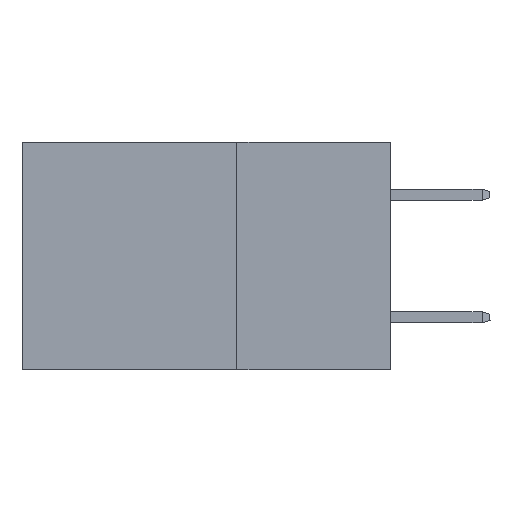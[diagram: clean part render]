
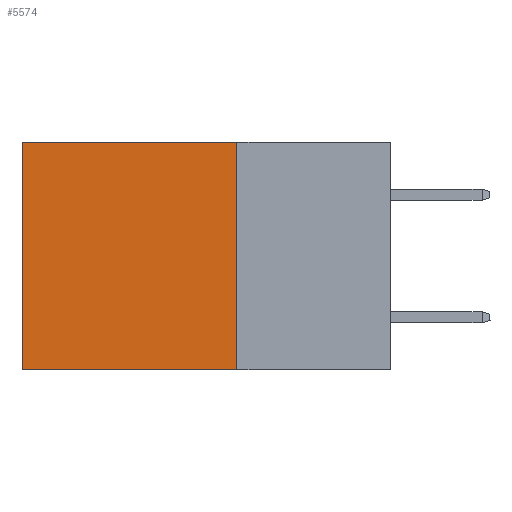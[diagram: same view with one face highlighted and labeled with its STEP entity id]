
A CAD part, left-side view. The second image highlights one B-rep face of the part: STEP entity #5574.
In plain terms, the highlighted planar face has unit normal (-1, 0, 0).
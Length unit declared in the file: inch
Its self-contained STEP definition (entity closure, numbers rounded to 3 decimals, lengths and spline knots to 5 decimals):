
#108 = LINE ( 'NONE', #9904, #724 ) ;
#724 = VECTOR ( 'NONE', #21830, 39.37008 ) ;
#992 = DIRECTION ( 'NONE',  ( 0., 1., 0. ) ) ;
#1916 = EDGE_CURVE ( 'NONE', #11666, #8930, #108, .T. ) ;
#2878 = EDGE_CURVE ( 'NONE', #23693, #8930, #4395, .T. ) ;
#3027 = ORIENTED_EDGE ( 'NONE', *, *, #3966, .F. ) ;
#3966 = EDGE_CURVE ( 'NONE', #14966, #23693, #5213, .T. ) ;
#4370 = EDGE_CURVE ( 'NONE', #14966, #11666, #19266, .T. ) ;
#4395 = LINE ( 'NONE', #18837, #23237 ) ;
#4481 = DIRECTION ( 'NONE',  ( 0., 0., -1. ) ) ;
#4634 = VECTOR ( 'NONE', #19960, 39.37008 ) ;
#5190 = VECTOR ( 'NONE', #992, 39.37008 ) ;
#5213 = LINE ( 'NONE', #11026, #4634 ) ;
#5574 = ADVANCED_FACE ( 'NONE', ( #22275 ), #8252, .F. ) ;
#6654 = CARTESIAN_POINT ( 'NONE',  ( 0.2875, 0.25, 0. ) ) ;
#8252 = PLANE ( 'NONE',  #16529 ) ;
#8254 = CARTESIAN_POINT ( 'NONE',  ( 0.2875, 0.6, -0.37 ) ) ;
#8930 = VERTEX_POINT ( 'NONE', #8254 ) ;
#9017 = CARTESIAN_POINT ( 'NONE',  ( 0.2875, 0.25, -0.37 ) ) ;
#9060 = ORIENTED_EDGE ( 'NONE', *, *, #1916, .T. ) ;
#9904 = CARTESIAN_POINT ( 'NONE',  ( 0.2875, 0.6, 0. ) ) ;
#10482 = EDGE_LOOP ( 'NONE', ( #9060, #11539, #3027, #12369 ) ) ;
#11026 = CARTESIAN_POINT ( 'NONE',  ( 0.2875, 0.25, 0. ) ) ;
#11539 = ORIENTED_EDGE ( 'NONE', *, *, #2878, .F. ) ;
#11666 = VERTEX_POINT ( 'NONE', #19236 ) ;
#12369 = ORIENTED_EDGE ( 'NONE', *, *, #4370, .T. ) ;
#13835 = CARTESIAN_POINT ( 'NONE',  ( 0.2875, 0.25, 0. ) ) ;
#14966 = VERTEX_POINT ( 'NONE', #19986 ) ;
#15626 = DIRECTION ( 'NONE',  ( 1., 0., 0. ) ) ;
#16529 = AXIS2_PLACEMENT_3D ( 'NONE', #13835, #15626, #4481 ) ;
#18837 = CARTESIAN_POINT ( 'NONE',  ( 0.2875, 0.25, -0.37 ) ) ;
#19236 = CARTESIAN_POINT ( 'NONE',  ( 0.2875, 0.6, 0. ) ) ;
#19266 = LINE ( 'NONE', #6654, #5190 ) ;
#19960 = DIRECTION ( 'NONE',  ( 0., 0., -1. ) ) ;
#19986 = CARTESIAN_POINT ( 'NONE',  ( 0.2875, 0.25, 0. ) ) ;
#20624 = DIRECTION ( 'NONE',  ( 0., 1., 0. ) ) ;
#21830 = DIRECTION ( 'NONE',  ( 0., 0., -1. ) ) ;
#22275 = FACE_OUTER_BOUND ( 'NONE', #10482, .T. ) ;
#23237 = VECTOR ( 'NONE', #20624, 39.37008 ) ;
#23693 = VERTEX_POINT ( 'NONE', #9017 ) ;
